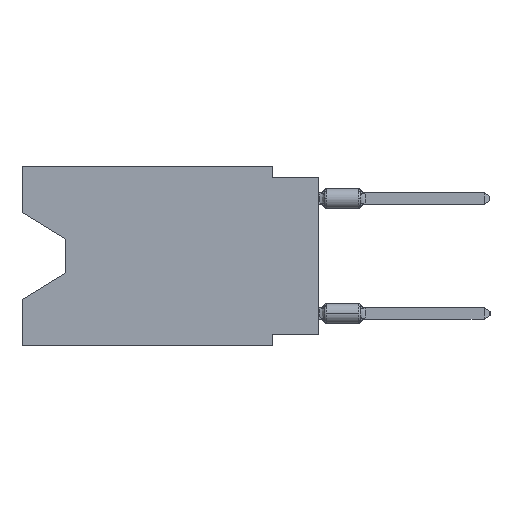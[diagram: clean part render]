
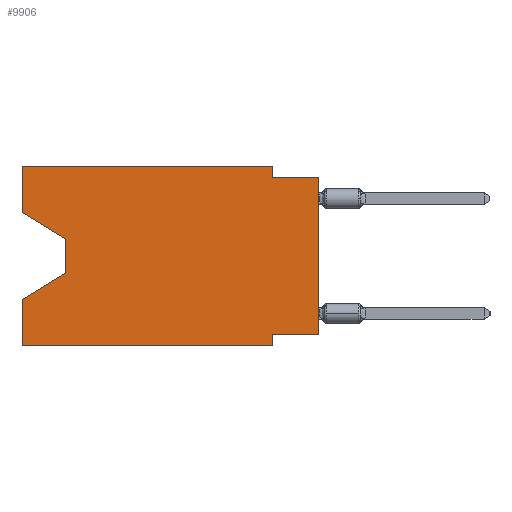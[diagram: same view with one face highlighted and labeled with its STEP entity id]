
A CAD part, left-side view. The second image highlights one B-rep face of the part: STEP entity #9906.
In plain terms, the highlighted planar face has unit normal (-1, 0, 0).
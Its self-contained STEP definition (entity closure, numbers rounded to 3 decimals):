
#1982 = CARTESIAN_POINT ( 'NONE',  ( 0., 0., -0.635 ) ) ;
#2202 = DIRECTION ( 'NONE',  ( 0., -0.855, -0.519 ) ) ;
#2285 = VERTEX_POINT ( 'NONE', #25204 ) ;
#2700 = VECTOR ( 'NONE', #28489, 1000. ) ;
#2900 = ORIENTED_EDGE ( 'NONE', *, *, #26033, .T. ) ;
#3985 = VECTOR ( 'NONE', #33248, 1000. ) ;
#4144 = CARTESIAN_POINT ( 'NONE',  ( 0., 16.383, -7.36 ) ) ;
#4929 = LINE ( 'NONE', #11349, #15745 ) ;
#5042 = EDGE_CURVE ( 'NONE', #36869, #32237, #6092, .T. ) ;
#5927 = DIRECTION ( 'NONE',  ( 0., 0., 1. ) ) ;
#6024 = VECTOR ( 'NONE', #5927, 1000. ) ;
#6092 = LINE ( 'NONE', #30599, #22415 ) ;
#6108 = DIRECTION ( 'NONE',  ( 0., 0., -1. ) ) ;
#6403 = EDGE_CURVE ( 'NONE', #25680, #20116, #19389, .T. ) ;
#7615 = VERTEX_POINT ( 'NONE', #20770 ) ;
#7666 = EDGE_CURVE ( 'NONE', #29033, #36571, #17667, .T. ) ;
#7746 = DIRECTION ( 'NONE',  ( 0., 0., 1. ) ) ;
#8140 = LINE ( 'NONE', #20593, #3985 ) ;
#8513 = VERTEX_POINT ( 'NONE', #1982 ) ;
#8883 = EDGE_CURVE ( 'NONE', #30218, #29033, #33073, .T. ) ;
#9029 = ORIENTED_EDGE ( 'NONE', *, *, #20294, .F. ) ;
#9230 = PLANE ( 'NONE',  #34876 ) ;
#9240 = CARTESIAN_POINT ( 'NONE',  ( 0., 16.383, 0. ) ) ;
#9252 = CARTESIAN_POINT ( 'NONE',  ( 0., 16.383, 0. ) ) ;
#9288 = CARTESIAN_POINT ( 'NONE',  ( 0., 16.383, -2.546 ) ) ;
#9906 = ADVANCED_FACE ( 'NONE', ( #21688 ), #9230, .F. ) ;
#10185 = CARTESIAN_POINT ( 'NONE',  ( 0., 2.54, -9.271 ) ) ;
#11210 = CARTESIAN_POINT ( 'NONE',  ( 0., 2.54, -9.906 ) ) ;
#11349 = CARTESIAN_POINT ( 'NONE',  ( 0., 16.383, -2.546 ) ) ;
#12014 = CARTESIAN_POINT ( 'NONE',  ( 0., 0., -0.635 ) ) ;
#12547 = ORIENTED_EDGE ( 'NONE', *, *, #6403, .T. ) ;
#13577 = VECTOR ( 'NONE', #15544, 1000. ) ;
#13664 = VERTEX_POINT ( 'NONE', #10185 ) ;
#14146 = DIRECTION ( 'NONE',  ( 0., 0.855, -0.519 ) ) ;
#14259 = LINE ( 'NONE', #36429, #40961 ) ;
#14387 = VECTOR ( 'NONE', #26867, 1000. ) ;
#15544 = DIRECTION ( 'NONE',  ( 0., -1., 0. ) ) ;
#15690 = EDGE_CURVE ( 'NONE', #25680, #36571, #27940, .T. ) ;
#15745 = VECTOR ( 'NONE', #2202, 1000. ) ;
#15840 = CARTESIAN_POINT ( 'NONE',  ( 0., 16.383, 0. ) ) ;
#16230 = VERTEX_POINT ( 'NONE', #29689 ) ;
#16721 = VECTOR ( 'NONE', #7746, 1000. ) ;
#17099 = LINE ( 'NONE', #30153, #16721 ) ;
#17165 = ORIENTED_EDGE ( 'NONE', *, *, #8883, .T. ) ;
#17655 = EDGE_CURVE ( 'NONE', #16230, #8513, #17099, .T. ) ;
#17667 = LINE ( 'NONE', #36921, #26265 ) ;
#18898 = VECTOR ( 'NONE', #30824, 1000. ) ;
#19389 = LINE ( 'NONE', #32030, #27986 ) ;
#19598 = DIRECTION ( 'NONE',  ( 0., -1., 0. ) ) ;
#19983 = CARTESIAN_POINT ( 'NONE',  ( 0., 13.97, -5.893 ) ) ;
#20116 = VERTEX_POINT ( 'NONE', #11210 ) ;
#20294 = EDGE_CURVE ( 'NONE', #7615, #8513, #37925, .T. ) ;
#20593 = CARTESIAN_POINT ( 'NONE',  ( 0., 2.54, -9.906 ) ) ;
#20770 = CARTESIAN_POINT ( 'NONE',  ( 0., 2.54, -0.635 ) ) ;
#21688 = FACE_OUTER_BOUND ( 'NONE', #24622, .T. ) ;
#22102 = CARTESIAN_POINT ( 'NONE',  ( 0., 16.383, 0. ) ) ;
#22415 = VECTOR ( 'NONE', #34118, 1000. ) ;
#24102 = ORIENTED_EDGE ( 'NONE', *, *, #26890, .F. ) ;
#24210 = CARTESIAN_POINT ( 'NONE',  ( 0., 0., -9.271 ) ) ;
#24622 = EDGE_LOOP ( 'NONE', ( #2900, #17165, #40702, #38783, #12547, #25616, #38356, #34632, #9029, #24102, #34923, #35809 ) ) ;
#24761 = EDGE_CURVE ( 'NONE', #16230, #13664, #30428, .T. ) ;
#25204 = CARTESIAN_POINT ( 'NONE',  ( 0., 2.54, 0. ) ) ;
#25616 = ORIENTED_EDGE ( 'NONE', *, *, #29070, .F. ) ;
#25680 = VERTEX_POINT ( 'NONE', #37712 ) ;
#26033 = EDGE_CURVE ( 'NONE', #36869, #30218, #4929, .T. ) ;
#26265 = VECTOR ( 'NONE', #14146, 1000. ) ;
#26867 = DIRECTION ( 'NONE',  ( 0., 0., -1. ) ) ;
#26890 = EDGE_CURVE ( 'NONE', #2285, #7615, #14259, .T. ) ;
#27940 = LINE ( 'NONE', #9252, #6024 ) ;
#27986 = VECTOR ( 'NONE', #19598, 1000. ) ;
#28489 = DIRECTION ( 'NONE',  ( 0., -1., 0. ) ) ;
#29033 = VERTEX_POINT ( 'NONE', #19983 ) ;
#29070 = EDGE_CURVE ( 'NONE', #13664, #20116, #8140, .T. ) ;
#29689 = CARTESIAN_POINT ( 'NONE',  ( 0., 0., -9.271 ) ) ;
#30008 = DIRECTION ( 'NONE',  ( 0., 0., -1. ) ) ;
#30114 = EDGE_CURVE ( 'NONE', #32237, #2285, #31582, .T. ) ;
#30153 = CARTESIAN_POINT ( 'NONE',  ( 0., 0., 0. ) ) ;
#30218 = VERTEX_POINT ( 'NONE', #35935 ) ;
#30428 = LINE ( 'NONE', #24210, #18898 ) ;
#30599 = CARTESIAN_POINT ( 'NONE',  ( 0., 16.383, 0. ) ) ;
#30824 = DIRECTION ( 'NONE',  ( 0., 1., 0. ) ) ;
#31582 = LINE ( 'NONE', #15840, #2700 ) ;
#32030 = CARTESIAN_POINT ( 'NONE',  ( 0., 16.383, -9.906 ) ) ;
#32237 = VERTEX_POINT ( 'NONE', #9240 ) ;
#33073 = LINE ( 'NONE', #36578, #14387 ) ;
#33248 = DIRECTION ( 'NONE',  ( 0., 0., -1. ) ) ;
#34118 = DIRECTION ( 'NONE',  ( 0., 0., 1. ) ) ;
#34632 = ORIENTED_EDGE ( 'NONE', *, *, #17655, .T. ) ;
#34876 = AXIS2_PLACEMENT_3D ( 'NONE', #22102, #37234, #6108 ) ;
#34923 = ORIENTED_EDGE ( 'NONE', *, *, #30114, .F. ) ;
#35809 = ORIENTED_EDGE ( 'NONE', *, *, #5042, .F. ) ;
#35935 = CARTESIAN_POINT ( 'NONE',  ( 0., 13.97, -4.013 ) ) ;
#36429 = CARTESIAN_POINT ( 'NONE',  ( 0., 2.54, 0. ) ) ;
#36571 = VERTEX_POINT ( 'NONE', #4144 ) ;
#36578 = CARTESIAN_POINT ( 'NONE',  ( 0., 13.97, -4.013 ) ) ;
#36869 = VERTEX_POINT ( 'NONE', #9288 ) ;
#36921 = CARTESIAN_POINT ( 'NONE',  ( 0., 13.97, -5.893 ) ) ;
#37234 = DIRECTION ( 'NONE',  ( 1., 0., 0. ) ) ;
#37712 = CARTESIAN_POINT ( 'NONE',  ( 0., 16.383, -9.906 ) ) ;
#37925 = LINE ( 'NONE', #12014, #13577 ) ;
#38356 = ORIENTED_EDGE ( 'NONE', *, *, #24761, .F. ) ;
#38783 = ORIENTED_EDGE ( 'NONE', *, *, #15690, .F. ) ;
#40702 = ORIENTED_EDGE ( 'NONE', *, *, #7666, .T. ) ;
#40961 = VECTOR ( 'NONE', #30008, 1000. ) ;
